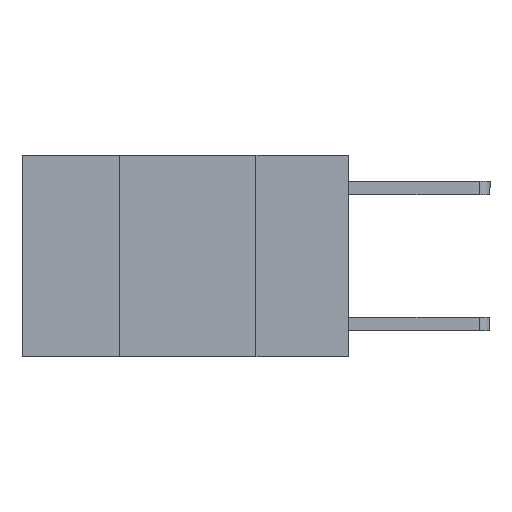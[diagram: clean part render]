
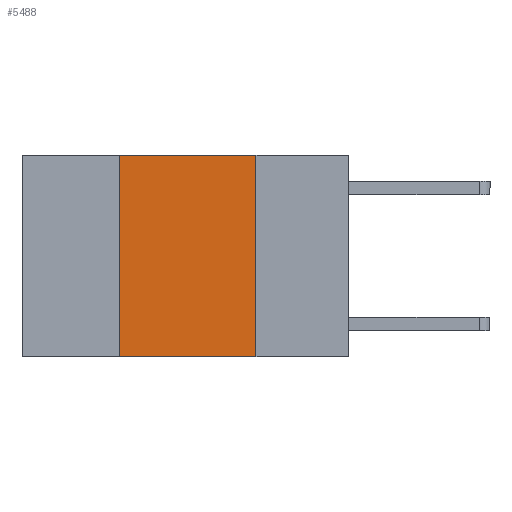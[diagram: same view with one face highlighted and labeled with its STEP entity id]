
A CAD part, left-side view. The second image highlights one B-rep face of the part: STEP entity #5488.
In plain terms, the highlighted planar face has unit normal (-1, 0, 0).
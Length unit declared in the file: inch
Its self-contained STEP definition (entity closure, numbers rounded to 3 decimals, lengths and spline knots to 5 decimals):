
#79 = EDGE_CURVE ( 'NONE', #130, #9698, #1422, .T. ) ;
#130 = VERTEX_POINT ( 'NONE', #9254 ) ;
#490 = CARTESIAN_POINT ( 'NONE',  ( 0., 0.42, 0. ) ) ;
#505 = ORIENTED_EDGE ( 'NONE', *, *, #5215, .F. ) ;
#585 = VECTOR ( 'NONE', #3402, 39.37008 ) ;
#951 = ORIENTED_EDGE ( 'NONE', *, *, #4330, .F. ) ;
#973 = VERTEX_POINT ( 'NONE', #5998 ) ;
#1422 = LINE ( 'NONE', #5985, #4274 ) ;
#2100 = DIRECTION ( 'NONE',  ( 0., -1., 0. ) ) ;
#2225 = VECTOR ( 'NONE', #9002, 39.37008 ) ;
#2539 = DIRECTION ( 'NONE',  ( 0., 0., -1. ) ) ;
#3402 = DIRECTION ( 'NONE',  ( 0., 0., -1. ) ) ;
#3914 = PLANE ( 'NONE',  #5966 ) ;
#4274 = VECTOR ( 'NONE', #4523, 39.37008 ) ;
#4330 = EDGE_CURVE ( 'NONE', #973, #9698, #5020, .T. ) ;
#4523 = DIRECTION ( 'NONE',  ( 0., -1., 0. ) ) ;
#5020 = LINE ( 'NONE', #5121, #585 ) ;
#5121 = CARTESIAN_POINT ( 'NONE',  ( 0., 0.17, 0. ) ) ;
#5215 = EDGE_CURVE ( 'NONE', #130, #8442, #7425, .T. ) ;
#5488 = ADVANCED_FACE ( 'NONE', ( #8784 ), #3914, .F. ) ;
#5526 = CARTESIAN_POINT ( 'NONE',  ( 0., 0.6, 0. ) ) ;
#5625 = DIRECTION ( 'NONE',  ( 1., 0., 0. ) ) ;
#5686 = ORIENTED_EDGE ( 'NONE', *, *, #8938, .F. ) ;
#5724 = CARTESIAN_POINT ( 'NONE',  ( 0., 0.42, 0. ) ) ;
#5952 = LINE ( 'NONE', #9063, #7979 ) ;
#5966 = AXIS2_PLACEMENT_3D ( 'NONE', #5526, #5625, #2539 ) ;
#5985 = CARTESIAN_POINT ( 'NONE',  ( 0., 0.6, -0.37 ) ) ;
#5998 = CARTESIAN_POINT ( 'NONE',  ( 0., 0.17, 0. ) ) ;
#6672 = EDGE_LOOP ( 'NONE', ( #951, #5686, #505, #9751 ) ) ;
#7425 = LINE ( 'NONE', #490, #2225 ) ;
#7979 = VECTOR ( 'NONE', #2100, 39.37008 ) ;
#8162 = CARTESIAN_POINT ( 'NONE',  ( 0., 0.17, -0.37 ) ) ;
#8442 = VERTEX_POINT ( 'NONE', #5724 ) ;
#8784 = FACE_OUTER_BOUND ( 'NONE', #6672, .T. ) ;
#8938 = EDGE_CURVE ( 'NONE', #8442, #973, #5952, .T. ) ;
#9002 = DIRECTION ( 'NONE',  ( 0., 0., 1. ) ) ;
#9063 = CARTESIAN_POINT ( 'NONE',  ( 0., 0.6, 0. ) ) ;
#9254 = CARTESIAN_POINT ( 'NONE',  ( 0., 0.42, -0.37 ) ) ;
#9698 = VERTEX_POINT ( 'NONE', #8162 ) ;
#9751 = ORIENTED_EDGE ( 'NONE', *, *, #79, .T. ) ;
